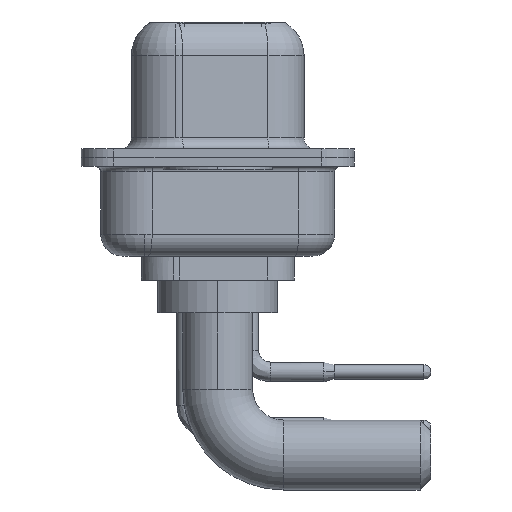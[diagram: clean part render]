
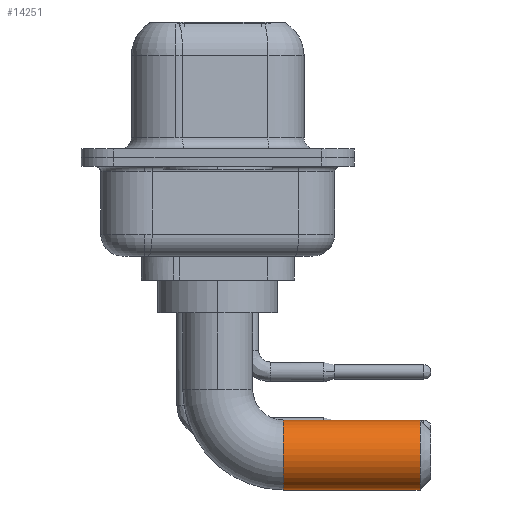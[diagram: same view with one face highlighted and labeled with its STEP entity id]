
A CAD part, left-side view. The second image highlights one B-rep face of the part: STEP entity #14251.
In plain terms, the highlighted cylindrical face has radius 1.6 mm (diameter 3.2 mm), a partial arc.
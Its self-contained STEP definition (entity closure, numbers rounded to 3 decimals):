
#19 = CARTESIAN_POINT ( 'NONE',  ( 0., -3., -4.9 ) ) ;
#227 = ORIENTED_EDGE ( 'NONE', *, *, #13162, .T. ) ;
#439 = EDGE_CURVE ( 'NONE', #15405, #6921, #15541, .T. ) ;
#724 = VERTEX_POINT ( 'NONE', #10790 ) ;
#743 = DIRECTION ( 'NONE',  ( 0., 0., -1. ) ) ;
#1519 = CARTESIAN_POINT ( 'NONE',  ( 0., -9.25, -6.5 ) ) ;
#1998 = FACE_OUTER_BOUND ( 'NONE', #16586, .T. ) ;
#2323 = CARTESIAN_POINT ( 'NONE',  ( 0., -3., -8.1 ) ) ;
#2399 = CARTESIAN_POINT ( 'NONE',  ( 0., -3., -6.5 ) ) ;
#3451 = CYLINDRICAL_SURFACE ( 'NONE', #9661, 1.6 ) ;
#3506 = VERTEX_POINT ( 'NONE', #5110 ) ;
#5110 = CARTESIAN_POINT ( 'NONE',  ( 0., -3., -4.9 ) ) ;
#5242 = ORIENTED_EDGE ( 'NONE', *, *, #439, .T. ) ;
#5537 = DIRECTION ( 'NONE',  ( 0., -1., 0. ) ) ;
#5614 = AXIS2_PLACEMENT_3D ( 'NONE', #1519, #15111, #11926 ) ;
#6447 = DIRECTION ( 'NONE',  ( 0., -1., 0. ) ) ;
#6921 = VERTEX_POINT ( 'NONE', #10048 ) ;
#7173 = CIRCLE ( 'NONE', #15491, 1.6 ) ;
#7298 = VECTOR ( 'NONE', #17065, 1000. ) ;
#8195 = DIRECTION ( 'NONE',  ( -1., 0., 0. ) ) ;
#8340 = EDGE_CURVE ( 'NONE', #3506, #724, #17369, .T. ) ;
#9661 = AXIS2_PLACEMENT_3D ( 'NONE', #15591, #6447, #743 ) ;
#10048 = CARTESIAN_POINT ( 'NONE',  ( 0., -9.25, -8.1 ) ) ;
#10597 = CARTESIAN_POINT ( 'NONE',  ( 0., -3., -8.1 ) ) ;
#10790 = CARTESIAN_POINT ( 'NONE',  ( 0., -9.25, -4.9 ) ) ;
#11627 = ORIENTED_EDGE ( 'NONE', *, *, #8340, .F. ) ;
#11926 = DIRECTION ( 'NONE',  ( 0., 0., -1. ) ) ;
#12067 = CIRCLE ( 'NONE', #5614, 1.6 ) ;
#13162 = EDGE_CURVE ( 'NONE', #6921, #724, #12067, .T. ) ;
#13471 = VECTOR ( 'NONE', #5537, 1000. ) ;
#13883 = EDGE_CURVE ( 'NONE', #3506, #15405, #7173, .T. ) ;
#14174 = DIRECTION ( 'NONE',  ( 0., -1., 0. ) ) ;
#14251 = ADVANCED_FACE ( 'NONE', ( #1998 ), #3451, .T. ) ;
#15111 = DIRECTION ( 'NONE',  ( 0., 1., 0. ) ) ;
#15195 = ORIENTED_EDGE ( 'NONE', *, *, #13883, .T. ) ;
#15405 = VERTEX_POINT ( 'NONE', #10597 ) ;
#15491 = AXIS2_PLACEMENT_3D ( 'NONE', #2399, #14174, #8195 ) ;
#15541 = LINE ( 'NONE', #2323, #7298 ) ;
#15591 = CARTESIAN_POINT ( 'NONE',  ( 0., -3., -6.5 ) ) ;
#16586 = EDGE_LOOP ( 'NONE', ( #11627, #15195, #5242, #227 ) ) ;
#17065 = DIRECTION ( 'NONE',  ( 0., -1., 0. ) ) ;
#17369 = LINE ( 'NONE', #19, #13471 ) ;
